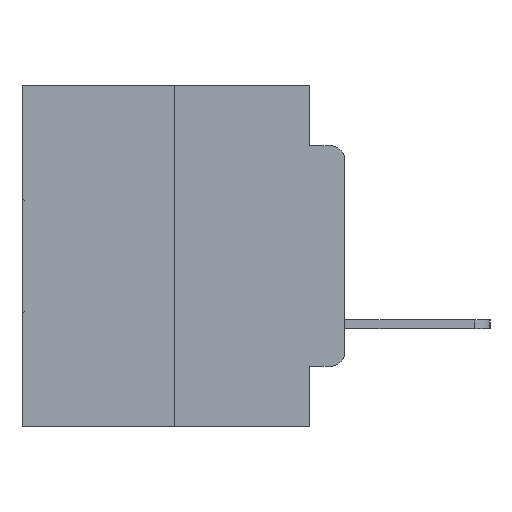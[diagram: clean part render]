
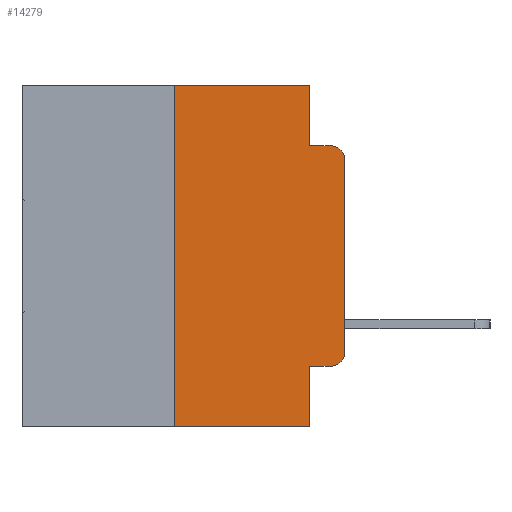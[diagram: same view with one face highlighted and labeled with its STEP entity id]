
A CAD part, left-side view. The second image highlights one B-rep face of the part: STEP entity #14279.
In plain terms, the highlighted planar face has unit normal (-1, 0, 0).
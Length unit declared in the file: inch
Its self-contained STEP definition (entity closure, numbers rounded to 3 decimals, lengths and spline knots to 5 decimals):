
#43 = CARTESIAN_POINT ( 'NONE',  ( 0., 0.25, 0. ) ) ;
#87 = DIRECTION ( 'NONE',  ( 0., 0., -1. ) ) ;
#169 = ORIENTED_EDGE ( 'NONE', *, *, #4726, .F. ) ;
#632 = DIRECTION ( 'NONE',  ( -1., 0., 0. ) ) ;
#788 = VECTOR ( 'NONE', #5330, 39.37008 ) ;
#1334 = VERTEX_POINT ( 'NONE', #23228 ) ;
#1465 = PLANE ( 'NONE',  #7346 ) ;
#1708 = VERTEX_POINT ( 'NONE', #23293 ) ;
#1716 = ORIENTED_EDGE ( 'NONE', *, *, #4768, .F. ) ;
#1726 = LINE ( 'NONE', #25133, #24164 ) ;
#1927 = CARTESIAN_POINT ( 'NONE',  ( 0., 0.02, -0.1085 ) ) ;
#2000 = VERTEX_POINT ( 'NONE', #43 ) ;
#2276 = VERTEX_POINT ( 'NONE', #24086 ) ;
#2556 = LINE ( 'NONE', #4537, #24871 ) ;
#3350 = EDGE_CURVE ( 'NONE', #2000, #14672, #19062, .T. ) ;
#3945 = DIRECTION ( 'NONE',  ( 0., 0., -1. ) ) ;
#4248 = EDGE_CURVE ( 'NONE', #1708, #12329, #2556, .T. ) ;
#4399 = DIRECTION ( 'NONE',  ( 0., 0., -1. ) ) ;
#4537 = CARTESIAN_POINT ( 'NONE',  ( 0., 0.473, -0.5 ) ) ;
#4597 = CARTESIAN_POINT ( 'NONE',  ( 0., 0.051, 0. ) ) ;
#4666 = EDGE_CURVE ( 'NONE', #5163, #1334, #9253, .T. ) ;
#4675 = EDGE_CURVE ( 'NONE', #1334, #24345, #15191, .T. ) ;
#4720 = EDGE_CURVE ( 'NONE', #12928, #24345, #13800, .T. ) ;
#4726 = EDGE_CURVE ( 'NONE', #14672, #12928, #7041, .T. ) ;
#4768 = EDGE_CURVE ( 'NONE', #1708, #2000, #11044, .T. ) ;
#4774 = EDGE_CURVE ( 'NONE', #2276, #12329, #10320, .T. ) ;
#4796 = ORIENTED_EDGE ( 'NONE', *, *, #4857, .T. ) ;
#4813 = VECTOR ( 'NONE', #87, 39.37008 ) ;
#4846 = CARTESIAN_POINT ( 'NONE',  ( 0., 0.02, -0.4115 ) ) ;
#4857 = EDGE_CURVE ( 'NONE', #2276, #7895, #1726, .T. ) ;
#4864 = EDGE_CURVE ( 'NONE', #7895, #5163, #6658, .T. ) ;
#5013 = CARTESIAN_POINT ( 'NONE',  ( 0., 0., -0.3915 ) ) ;
#5163 = VERTEX_POINT ( 'NONE', #5013 ) ;
#5330 = DIRECTION ( 'NONE',  ( 0., -1., 0. ) ) ;
#6264 = CARTESIAN_POINT ( 'NONE',  ( 0., 0.473, 0. ) ) ;
#6646 = ORIENTED_EDGE ( 'NONE', *, *, #3350, .F. ) ;
#6658 = CIRCLE ( 'NONE', #8304, 0.02 ) ;
#6931 = DIRECTION ( 'NONE',  ( 0., -1., 0. ) ) ;
#7041 = LINE ( 'NONE', #4597, #12454 ) ;
#7346 = AXIS2_PLACEMENT_3D ( 'NONE', #6264, #13171, #3945 ) ;
#7895 = VERTEX_POINT ( 'NONE', #4846 ) ;
#8304 = AXIS2_PLACEMENT_3D ( 'NONE', #14622, #632, #16803 ) ;
#9253 = LINE ( 'NONE', #24059, #25783 ) ;
#10320 = LINE ( 'NONE', #16336, #4813 ) ;
#11044 = LINE ( 'NONE', #17375, #16204 ) ;
#11439 = CARTESIAN_POINT ( 'NONE',  ( 0., 0.051, -0.5 ) ) ;
#11467 = DIRECTION ( 'NONE',  ( 0., -1., 0. ) ) ;
#11626 = CARTESIAN_POINT ( 'NONE',  ( 0., 0.051, -0.0885 ) ) ;
#12329 = VERTEX_POINT ( 'NONE', #11439 ) ;
#12337 = DIRECTION ( 'NONE',  ( 0., -1., 0. ) ) ;
#12454 = VECTOR ( 'NONE', #18146, 39.37008 ) ;
#12928 = VERTEX_POINT ( 'NONE', #11626 ) ;
#13115 = VECTOR ( 'NONE', #11467, 39.37008 ) ;
#13171 = DIRECTION ( 'NONE',  ( 1., 0., 0. ) ) ;
#13800 = LINE ( 'NONE', #22295, #13115 ) ;
#14052 = DIRECTION ( 'NONE',  ( 0., 0., 1. ) ) ;
#14279 = ADVANCED_FACE ( 'NONE', ( #18005 ), #1465, .F. ) ;
#14622 = CARTESIAN_POINT ( 'NONE',  ( 0., 0.02, -0.3915 ) ) ;
#14672 = VERTEX_POINT ( 'NONE', #20887 ) ;
#15191 = CIRCLE ( 'NONE', #28187, 0.02 ) ;
#16194 = ORIENTED_EDGE ( 'NONE', *, *, #4774, .F. ) ;
#16204 = VECTOR ( 'NONE', #14052, 39.37008 ) ;
#16336 = CARTESIAN_POINT ( 'NONE',  ( 0., 0.051, 0. ) ) ;
#16511 = ORIENTED_EDGE ( 'NONE', *, *, #4720, .F. ) ;
#16803 = DIRECTION ( 'NONE',  ( 0., 0., -1. ) ) ;
#17375 = CARTESIAN_POINT ( 'NONE',  ( 0., 0.25, 0. ) ) ;
#17952 = DIRECTION ( 'NONE',  ( -1., 0., 0. ) ) ;
#18005 = FACE_OUTER_BOUND ( 'NONE', #18502, .T. ) ;
#18146 = DIRECTION ( 'NONE',  ( 0., 0., -1. ) ) ;
#18502 = EDGE_LOOP ( 'NONE', ( #20510, #20855, #16511, #169, #6646, #1716, #25446, #16194, #4796, #28707 ) ) ;
#19062 = LINE ( 'NONE', #23010, #788 ) ;
#20510 = ORIENTED_EDGE ( 'NONE', *, *, #4666, .T. ) ;
#20855 = ORIENTED_EDGE ( 'NONE', *, *, #4675, .T. ) ;
#20887 = CARTESIAN_POINT ( 'NONE',  ( 0., 0.051, 0. ) ) ;
#22295 = CARTESIAN_POINT ( 'NONE',  ( 0., 0.051, -0.0885 ) ) ;
#23010 = CARTESIAN_POINT ( 'NONE',  ( 0., 0.473, 0. ) ) ;
#23228 = CARTESIAN_POINT ( 'NONE',  ( 0., 0., -0.1085 ) ) ;
#23293 = CARTESIAN_POINT ( 'NONE',  ( 0., 0.25, -0.5 ) ) ;
#24059 = CARTESIAN_POINT ( 'NONE',  ( 0., 0., 0. ) ) ;
#24086 = CARTESIAN_POINT ( 'NONE',  ( 0., 0.051, -0.4115 ) ) ;
#24164 = VECTOR ( 'NONE', #12337, 39.37008 ) ;
#24345 = VERTEX_POINT ( 'NONE', #25716 ) ;
#24871 = VECTOR ( 'NONE', #6931, 39.37008 ) ;
#25133 = CARTESIAN_POINT ( 'NONE',  ( 0., 0.051, -0.4115 ) ) ;
#25446 = ORIENTED_EDGE ( 'NONE', *, *, #4248, .T. ) ;
#25716 = CARTESIAN_POINT ( 'NONE',  ( 0., 0.02, -0.0885 ) ) ;
#25783 = VECTOR ( 'NONE', #26218, 39.37008 ) ;
#26218 = DIRECTION ( 'NONE',  ( 0., 0., 1. ) ) ;
#28187 = AXIS2_PLACEMENT_3D ( 'NONE', #1927, #17952, #4399 ) ;
#28707 = ORIENTED_EDGE ( 'NONE', *, *, #4864, .T. ) ;
